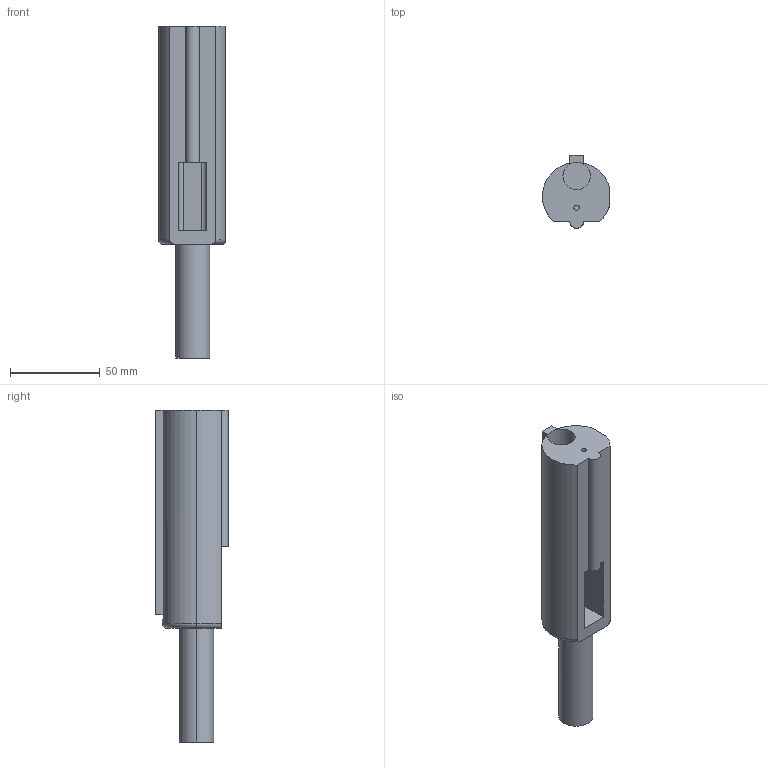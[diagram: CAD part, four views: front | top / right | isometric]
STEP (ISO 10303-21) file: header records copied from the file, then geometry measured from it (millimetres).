
FILE_DESCRIPTION (( 'STEP AP214' ), '1' );
FILE_NAME ('bolt.STEP', '2013-11-06T01:52:16', ( '' ), ( '' ), 'SwSTEP 2.0', 'SolidWorks 2013', '' );
FILE_SCHEMA (( 'AUTOMOTIVE_DESIGN' ));
Length unit declared in the file: inch
Products named in the file (1): bolt
Bounding box: 37.39 x 40.64 x 185.42 mm (x, y, z)
Volume: 114062.5 mm3; surface area: 31343.5 mm2
Topology: 1 solids, 1 shells, 44 faces, 107 edges, 71 vertices
Faces by surface type: plane 23, cylinder 18, torus 3
Entity records: 1412 total; most frequent: CARTESIAN_POINT 293, DIRECTION 236, ORIENTED_EDGE 214, EDGE_CURVE 107, AXIS2_PLACEMENT_3D 88, VERTEX_POINT 71, VECTOR 60, LINE 60
